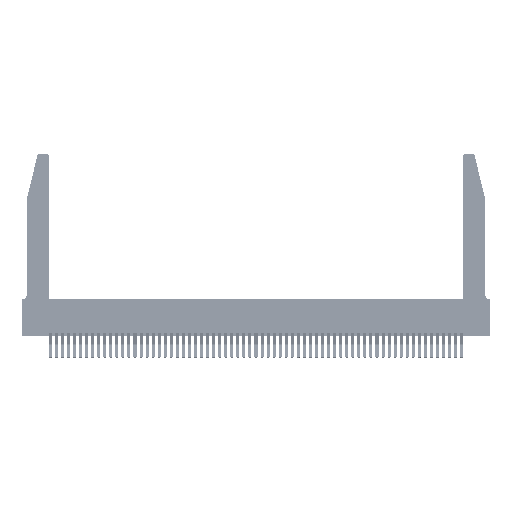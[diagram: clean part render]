
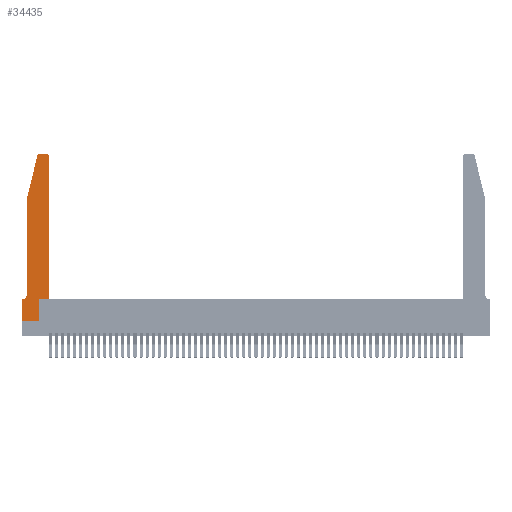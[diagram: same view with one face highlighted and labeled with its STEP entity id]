
A CAD part, top view. The second image highlights one B-rep face of the part: STEP entity #34435.
In plain terms, the highlighted planar face has unit normal (0, 0, 1).
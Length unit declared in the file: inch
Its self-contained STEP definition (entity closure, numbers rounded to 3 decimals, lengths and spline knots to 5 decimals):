
#50 = LINE ( 'NONE', #14145, #50235 ) ;
#353 = VERTEX_POINT ( 'NONE', #889 ) ;
#443 = CARTESIAN_POINT ( 'NONE',  ( 0.0755, 2., 0.37 ) ) ;
#610 = EDGE_CURVE ( 'NONE', #353, #51729, #29609, .T. ) ;
#889 = CARTESIAN_POINT ( 'NONE',  ( 0.2865, 0., 0.37 ) ) ;
#2088 = CARTESIAN_POINT ( 'NONE',  ( 0.0755, 0.35, 0.37 ) ) ;
#2494 = EDGE_CURVE ( 'NONE', #15128, #39521, #5502, .T. ) ;
#2903 = ORIENTED_EDGE ( 'NONE', *, *, #40450, .T. ) ;
#3561 = ORIENTED_EDGE ( 'NONE', *, *, #41760, .T. ) ;
#3872 = VERTEX_POINT ( 'NONE', #16720 ) ;
#3926 = CARTESIAN_POINT ( 'NONE',  ( 0.4505, 0.35, 0.37 ) ) ;
#4198 = CARTESIAN_POINT ( 'NONE',  ( 0., 0.35, 0.37 ) ) ;
#4581 = VECTOR ( 'NONE', #25911, 39.37008 ) ;
#5277 = FACE_OUTER_BOUND ( 'NONE', #5865, .T. ) ;
#5502 = CIRCLE ( 'NONE', #12141, 0.03 ) ;
#5865 = EDGE_LOOP ( 'NONE', ( #18226, #6106, #27092, #22754, #3561, #10294, #6087, #33326, #13662, #10576, #2903, #45167 ) ) ;
#6087 = ORIENTED_EDGE ( 'NONE', *, *, #13840, .T. ) ;
#6106 = ORIENTED_EDGE ( 'NONE', *, *, #2494, .T. ) ;
#6897 = CARTESIAN_POINT ( 'NONE',  ( 0.284, 2.72, 0.37 ) ) ;
#7412 = DIRECTION ( 'NONE',  ( 0., 0., 1. ) ) ;
#7494 = AXIS2_PLACEMENT_3D ( 'NONE', #4198, #34565, #34752 ) ;
#7571 = CARTESIAN_POINT ( 'NONE',  ( 0.0055, 0.42, 0.37 ) ) ;
#9512 = CARTESIAN_POINT ( 'NONE',  ( 0.0055, 0.35, 0.37 ) ) ;
#10294 = ORIENTED_EDGE ( 'NONE', *, *, #48550, .T. ) ;
#10576 = ORIENTED_EDGE ( 'NONE', *, *, #17364, .T. ) ;
#10896 = CARTESIAN_POINT ( 'NONE',  ( 0.0755, 0.42, 0.37 ) ) ;
#11027 = EDGE_CURVE ( 'NONE', #14461, #15128, #50, .T. ) ;
#12141 = AXIS2_PLACEMENT_3D ( 'NONE', #6897, #15561, #45490 ) ;
#12277 = LINE ( 'NONE', #55030, #29624 ) ;
#12590 = EDGE_CURVE ( 'NONE', #39521, #26727, #51488, .T. ) ;
#12596 = EDGE_CURVE ( 'NONE', #26727, #12859, #40770, .T. ) ;
#12859 = VERTEX_POINT ( 'NONE', #10896 ) ;
#13250 = CARTESIAN_POINT ( 'NONE',  ( 0.4505, 2.72, 0.37 ) ) ;
#13420 = AXIS2_PLACEMENT_3D ( 'NONE', #41129, #7412, #46159 ) ;
#13662 = ORIENTED_EDGE ( 'NONE', *, *, #610, .T. ) ;
#13840 = EDGE_CURVE ( 'NONE', #3872, #41079, #47977, .T. ) ;
#14145 = CARTESIAN_POINT ( 'NONE',  ( 0.2605, 2.75, 0.37 ) ) ;
#14461 = VERTEX_POINT ( 'NONE', #54314 ) ;
#14678 = VECTOR ( 'NONE', #34709, 39.37008 ) ;
#15128 = VERTEX_POINT ( 'NONE', #34446 ) ;
#15561 = DIRECTION ( 'NONE',  ( 0., 0., 1. ) ) ;
#16125 = DIRECTION ( 'NONE',  ( -1., 0., 0. ) ) ;
#16720 = CARTESIAN_POINT ( 'NONE',  ( 0., 0.35, 0.37 ) ) ;
#16970 = PLANE ( 'NONE',  #7494 ) ;
#17364 = EDGE_CURVE ( 'NONE', #51729, #25982, #12277, .T. ) ;
#17482 = CARTESIAN_POINT ( 'NONE',  ( 0.0755, 2., 0.37 ) ) ;
#18226 = ORIENTED_EDGE ( 'NONE', *, *, #11027, .T. ) ;
#18330 = CARTESIAN_POINT ( 'NONE',  ( 0.25487, 2.72718, 0.37 ) ) ;
#19584 = EDGE_CURVE ( 'NONE', #41079, #353, #47584, .T. ) ;
#20518 = DIRECTION ( 'NONE',  ( 0., 0., -1. ) ) ;
#21406 = DIRECTION ( 'NONE',  ( 0., 1., 0. ) ) ;
#22040 = DIRECTION ( 'NONE',  ( 0., -1., 0. ) ) ;
#22754 = ORIENTED_EDGE ( 'NONE', *, *, #12596, .T. ) ;
#24335 = VECTOR ( 'NONE', #21406, 39.37008 ) ;
#25911 = DIRECTION ( 'NONE',  ( 0., -1., 0. ) ) ;
#25982 = VERTEX_POINT ( 'NONE', #32783 ) ;
#26727 = VERTEX_POINT ( 'NONE', #17482 ) ;
#27092 = ORIENTED_EDGE ( 'NONE', *, *, #12590, .T. ) ;
#28935 = CARTESIAN_POINT ( 'NONE',  ( 0.2865, 0.35, 0.37 ) ) ;
#29459 = DIRECTION ( 'NONE',  ( 1., 0., 0. ) ) ;
#29609 = LINE ( 'NONE', #28935, #50312 ) ;
#29624 = VECTOR ( 'NONE', #29459, 39.37008 ) ;
#32783 = CARTESIAN_POINT ( 'NONE',  ( 0.4505, 0.35, 0.37 ) ) ;
#32960 = CARTESIAN_POINT ( 'NONE',  ( 0., 0., 0.37 ) ) ;
#33326 = ORIENTED_EDGE ( 'NONE', *, *, #19584, .T. ) ;
#33367 = CIRCLE ( 'NONE', #52518, 0.07 ) ;
#33440 = DIRECTION ( 'NONE',  ( -1., 0., 0. ) ) ;
#33643 = LINE ( 'NONE', #2088, #38996 ) ;
#34435 = ADVANCED_FACE ( 'NONE', ( #5277 ), #16970, .T. ) ;
#34446 = CARTESIAN_POINT ( 'NONE',  ( 0.284, 2.75, 0.37 ) ) ;
#34565 = DIRECTION ( 'NONE',  ( 0., 0., 1. ) ) ;
#34709 = DIRECTION ( 'NONE',  ( -0.239, -0.971, 0. ) ) ;
#34752 = DIRECTION ( 'NONE',  ( 1., 0., 0. ) ) ;
#35116 = DIRECTION ( 'NONE',  ( -1., 0., 0. ) ) ;
#36527 = DIRECTION ( 'NONE',  ( 1., 0., 0. ) ) ;
#37359 = DIRECTION ( 'NONE',  ( 0., 1., 0. ) ) ;
#38996 = VECTOR ( 'NONE', #16125, 39.37008 ) ;
#39275 = VECTOR ( 'NONE', #22040, 39.37008 ) ;
#39521 = VERTEX_POINT ( 'NONE', #18330 ) ;
#40450 = EDGE_CURVE ( 'NONE', #25982, #49495, #46385, .T. ) ;
#40770 = LINE ( 'NONE', #443, #4581 ) ;
#41079 = VERTEX_POINT ( 'NONE', #32960 ) ;
#41129 = CARTESIAN_POINT ( 'NONE',  ( 0.4205, 2.72, 0.37 ) ) ;
#41760 = EDGE_CURVE ( 'NONE', #12859, #49454, #33367, .T. ) ;
#44409 = CARTESIAN_POINT ( 'NONE',  ( 0.2865, 0.35, 0.37 ) ) ;
#44774 = CARTESIAN_POINT ( 'NONE',  ( 0., 0., 0.37 ) ) ;
#45167 = ORIENTED_EDGE ( 'NONE', *, *, #52568, .T. ) ;
#45490 = DIRECTION ( 'NONE',  ( 1., 0., 0. ) ) ;
#46159 = DIRECTION ( 'NONE',  ( 1., 0., 0. ) ) ;
#46385 = LINE ( 'NONE', #3926, #24335 ) ;
#47285 = CARTESIAN_POINT ( 'NONE',  ( 0., 0., 0.37 ) ) ;
#47584 = LINE ( 'NONE', #44774, #53564 ) ;
#47617 = CARTESIAN_POINT ( 'NONE',  ( 0.0755, 2., 0.37 ) ) ;
#47977 = LINE ( 'NONE', #47285, #39275 ) ;
#48550 = EDGE_CURVE ( 'NONE', #49454, #3872, #33643, .T. ) ;
#49454 = VERTEX_POINT ( 'NONE', #9512 ) ;
#49495 = VERTEX_POINT ( 'NONE', #13250 ) ;
#50235 = VECTOR ( 'NONE', #35116, 39.37008 ) ;
#50312 = VECTOR ( 'NONE', #37359, 39.37008 ) ;
#51215 = CIRCLE ( 'NONE', #13420, 0.03 ) ;
#51488 = LINE ( 'NONE', #47617, #14678 ) ;
#51729 = VERTEX_POINT ( 'NONE', #44409 ) ;
#52518 = AXIS2_PLACEMENT_3D ( 'NONE', #7571, #20518, #33440 ) ;
#52568 = EDGE_CURVE ( 'NONE', #49495, #14461, #51215, .T. ) ;
#53564 = VECTOR ( 'NONE', #36527, 39.37008 ) ;
#54314 = CARTESIAN_POINT ( 'NONE',  ( 0.4205, 2.75, 0.37 ) ) ;
#55030 = CARTESIAN_POINT ( 'NONE',  ( 0.4505, 0.35, 0.37 ) ) ;
